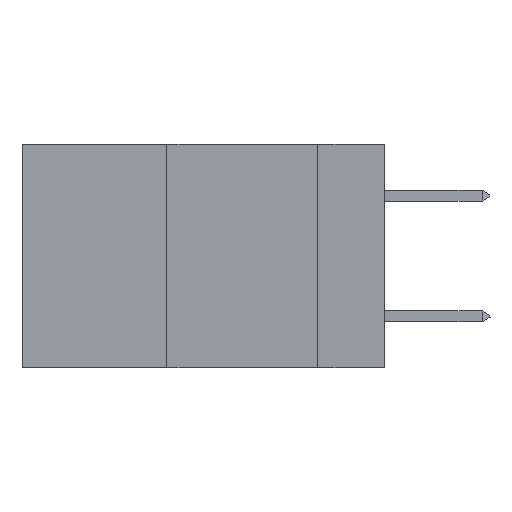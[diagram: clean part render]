
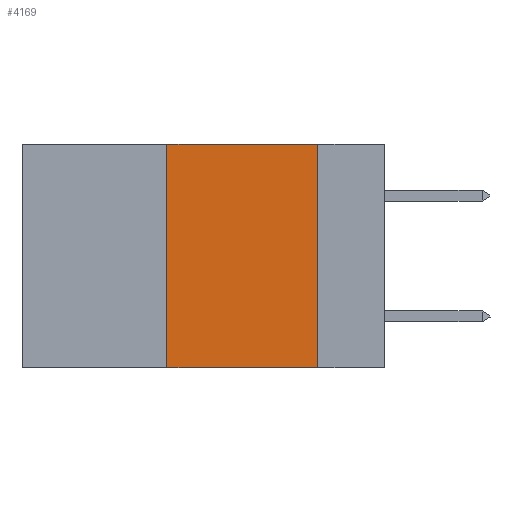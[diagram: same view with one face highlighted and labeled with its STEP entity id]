
A CAD part, left-side view. The second image highlights one B-rep face of the part: STEP entity #4169.
In plain terms, the highlighted planar face has unit normal (-1, 0, 0).
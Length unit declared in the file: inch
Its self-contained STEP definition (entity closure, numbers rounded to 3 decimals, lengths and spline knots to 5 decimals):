
#223 = EDGE_CURVE ( 'NONE', #7381, #12582, #8125, .T. ) ;
#258 = CARTESIAN_POINT ( 'NONE',  ( 0., 0.36, 0. ) ) ;
#538 = AXIS2_PLACEMENT_3D ( 'NONE', #6553, #9882, #773 ) ;
#773 = DIRECTION ( 'NONE',  ( 0., 0., -1. ) ) ;
#2038 = DIRECTION ( 'NONE',  ( 0., -1., 0. ) ) ;
#2164 = ORIENTED_EDGE ( 'NONE', *, *, #6766, .F. ) ;
#2463 = EDGE_CURVE ( 'NONE', #4526, #12582, #6199, .T. ) ;
#2476 = DIRECTION ( 'NONE',  ( 0., -1., 0. ) ) ;
#2580 = FACE_OUTER_BOUND ( 'NONE', #5755, .T. ) ;
#2861 = LINE ( 'NONE', #12221, #3014 ) ;
#3014 = VECTOR ( 'NONE', #12347, 39.37008 ) ;
#3913 = CARTESIAN_POINT ( 'NONE',  ( 0., 0.36, -0.37 ) ) ;
#4169 = ADVANCED_FACE ( 'NONE', ( #2580 ), #7514, .F. ) ;
#4526 = VERTEX_POINT ( 'NONE', #3913 ) ;
#5400 = VECTOR ( 'NONE', #2476, 39.37008 ) ;
#5755 = EDGE_LOOP ( 'NONE', ( #7805, #7692, #2164, #9264 ) ) ;
#5894 = DIRECTION ( 'NONE',  ( 0., 0., -1. ) ) ;
#6199 = LINE ( 'NONE', #6426, #5400 ) ;
#6256 = CARTESIAN_POINT ( 'NONE',  ( 0., 0.6, 0. ) ) ;
#6426 = CARTESIAN_POINT ( 'NONE',  ( 0., 0.6, -0.37 ) ) ;
#6553 = CARTESIAN_POINT ( 'NONE',  ( 0., 0.6, 0. ) ) ;
#6766 = EDGE_CURVE ( 'NONE', #4526, #8269, #2861, .T. ) ;
#7251 = CARTESIAN_POINT ( 'NONE',  ( 0., 0.11, 0. ) ) ;
#7381 = VERTEX_POINT ( 'NONE', #7251 ) ;
#7514 = PLANE ( 'NONE',  #538 ) ;
#7692 = ORIENTED_EDGE ( 'NONE', *, *, #11623, .F. ) ;
#7805 = ORIENTED_EDGE ( 'NONE', *, *, #223, .F. ) ;
#8125 = LINE ( 'NONE', #10671, #11596 ) ;
#8269 = VERTEX_POINT ( 'NONE', #258 ) ;
#8780 = VECTOR ( 'NONE', #2038, 39.37008 ) ;
#8953 = LINE ( 'NONE', #6256, #8780 ) ;
#9264 = ORIENTED_EDGE ( 'NONE', *, *, #2463, .T. ) ;
#9882 = DIRECTION ( 'NONE',  ( 1., 0., 0. ) ) ;
#10347 = CARTESIAN_POINT ( 'NONE',  ( 0., 0.11, -0.37 ) ) ;
#10671 = CARTESIAN_POINT ( 'NONE',  ( 0., 0.11, 0. ) ) ;
#11596 = VECTOR ( 'NONE', #5894, 39.37008 ) ;
#11623 = EDGE_CURVE ( 'NONE', #8269, #7381, #8953, .T. ) ;
#12221 = CARTESIAN_POINT ( 'NONE',  ( 0., 0.36, 0. ) ) ;
#12347 = DIRECTION ( 'NONE',  ( 0., 0., 1. ) ) ;
#12582 = VERTEX_POINT ( 'NONE', #10347 ) ;
